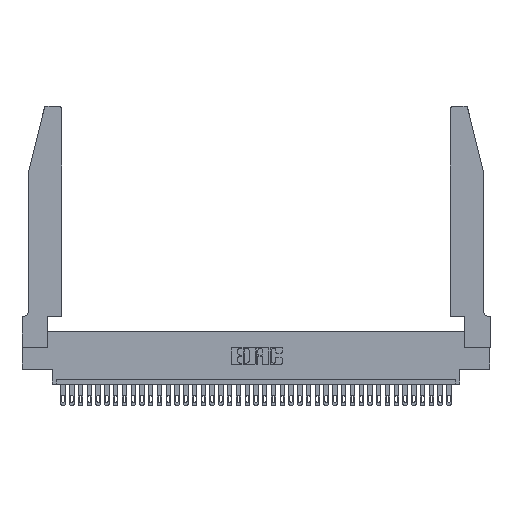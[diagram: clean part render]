
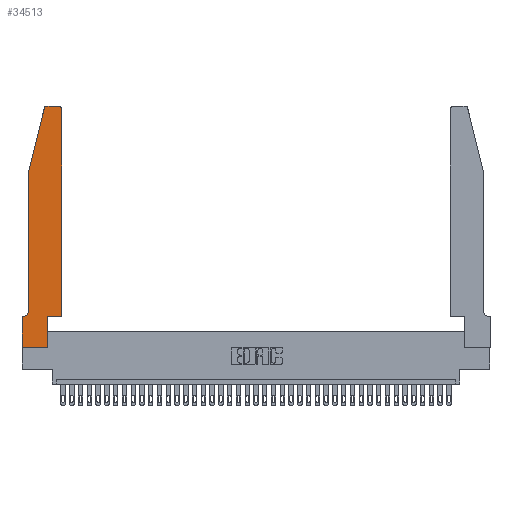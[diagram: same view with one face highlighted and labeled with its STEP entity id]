
A CAD part, top view. The second image highlights one B-rep face of the part: STEP entity #34513.
In plain terms, the highlighted planar face has unit normal (0, 0, 1).
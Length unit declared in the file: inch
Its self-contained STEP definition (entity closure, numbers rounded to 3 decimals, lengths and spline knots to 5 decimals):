
#97 = VERTEX_POINT ( 'NONE', #2483 ) ;
#175 = CARTESIAN_POINT ( 'NONE',  ( 0.0755, 2., 0.37 ) ) ;
#212 = CARTESIAN_POINT ( 'NONE',  ( 0.284, 2.72, 0.37 ) ) ;
#771 = VERTEX_POINT ( 'NONE', #37358 ) ;
#863 = CARTESIAN_POINT ( 'NONE',  ( 0.0755, 0.42, 0.37 ) ) ;
#1432 = EDGE_CURVE ( 'NONE', #24707, #26314, #30907, .T. ) ;
#2483 = CARTESIAN_POINT ( 'NONE',  ( 0.2865, 0.35, 0.37 ) ) ;
#2685 = EDGE_CURVE ( 'NONE', #26314, #23081, #18780, .T. ) ;
#3274 = ORIENTED_EDGE ( 'NONE', *, *, #8241, .T. ) ;
#3347 = CIRCLE ( 'NONE', #3746, 0.07 ) ;
#3746 = AXIS2_PLACEMENT_3D ( 'NONE', #6014, #6139, #11941 ) ;
#3758 = CARTESIAN_POINT ( 'NONE',  ( 0.2865, 0.35, 0.37 ) ) ;
#4425 = DIRECTION ( 'NONE',  ( 0., 1., 0. ) ) ;
#4665 = CARTESIAN_POINT ( 'NONE',  ( 0.4205, 2.75, 0.37 ) ) ;
#4867 = VERTEX_POINT ( 'NONE', #12759 ) ;
#5276 = CARTESIAN_POINT ( 'NONE',  ( 0., 0., 0.37 ) ) ;
#5482 = CARTESIAN_POINT ( 'NONE',  ( 0.25487, 2.72718, 0.37 ) ) ;
#6014 = CARTESIAN_POINT ( 'NONE',  ( 0.0055, 0.42, 0.37 ) ) ;
#6139 = DIRECTION ( 'NONE',  ( 0., 0., -1. ) ) ;
#6354 = VECTOR ( 'NONE', #14589, 39.37008 ) ;
#7670 = ORIENTED_EDGE ( 'NONE', *, *, #2685, .T. ) ;
#8241 = EDGE_CURVE ( 'NONE', #9883, #97, #9208, .T. ) ;
#8861 = ORIENTED_EDGE ( 'NONE', *, *, #19691, .T. ) ;
#9193 = DIRECTION ( 'NONE',  ( 0., 1., 0. ) ) ;
#9208 = LINE ( 'NONE', #3758, #34604 ) ;
#9423 = VECTOR ( 'NONE', #26111, 39.37008 ) ;
#9756 = ORIENTED_EDGE ( 'NONE', *, *, #19706, .T. ) ;
#9883 = VERTEX_POINT ( 'NONE', #12087 ) ;
#10145 = VECTOR ( 'NONE', #11916, 39.37008 ) ;
#10898 = DIRECTION ( 'NONE',  ( 0., 0., 1. ) ) ;
#11292 = CARTESIAN_POINT ( 'NONE',  ( 0.0755, 2., 0.37 ) ) ;
#11916 = DIRECTION ( 'NONE',  ( 0., -1., 0. ) ) ;
#11941 = DIRECTION ( 'NONE',  ( -1., 0., 0. ) ) ;
#12087 = CARTESIAN_POINT ( 'NONE',  ( 0.2865, 0., 0.37 ) ) ;
#12759 = CARTESIAN_POINT ( 'NONE',  ( 0., 0.35, 0.37 ) ) ;
#13321 = ORIENTED_EDGE ( 'NONE', *, *, #31277, .T. ) ;
#13360 = LINE ( 'NONE', #175, #10145 ) ;
#13736 = DIRECTION ( 'NONE',  ( 1., 0., 0. ) ) ;
#13812 = ORIENTED_EDGE ( 'NONE', *, *, #15193, .T. ) ;
#14589 = DIRECTION ( 'NONE',  ( 1., 0., 0. ) ) ;
#14702 = VERTEX_POINT ( 'NONE', #17727 ) ;
#14715 = FACE_OUTER_BOUND ( 'NONE', #21656, .T. ) ;
#15193 = EDGE_CURVE ( 'NONE', #23081, #16428, #13360, .T. ) ;
#15401 = CARTESIAN_POINT ( 'NONE',  ( 0., 0.35, 0.37 ) ) ;
#15605 = ORIENTED_EDGE ( 'NONE', *, *, #25438, .T. ) ;
#16428 = VERTEX_POINT ( 'NONE', #863 ) ;
#17727 = CARTESIAN_POINT ( 'NONE',  ( 0.0055, 0.35, 0.37 ) ) ;
#18396 = ORIENTED_EDGE ( 'NONE', *, *, #26589, .T. ) ;
#18499 = DIRECTION ( 'NONE',  ( 1., 0., 0. ) ) ;
#18740 = CARTESIAN_POINT ( 'NONE',  ( 0., 0., 0.37 ) ) ;
#18780 = LINE ( 'NONE', #23416, #28484 ) ;
#19011 = ORIENTED_EDGE ( 'NONE', *, *, #21983, .T. ) ;
#19507 = AXIS2_PLACEMENT_3D ( 'NONE', #15401, #24183, #30630 ) ;
#19691 = EDGE_CURVE ( 'NONE', #4867, #32729, #24784, .T. ) ;
#19706 = EDGE_CURVE ( 'NONE', #771, #23542, #29541, .T. ) ;
#20011 = CIRCLE ( 'NONE', #24924, 0.03 ) ;
#20039 = EDGE_CURVE ( 'NONE', #97, #771, #37313, .T. ) ;
#20171 = CARTESIAN_POINT ( 'NONE',  ( 0.2605, 2.75, 0.37 ) ) ;
#20582 = VECTOR ( 'NONE', #33196, 39.37008 ) ;
#20840 = ORIENTED_EDGE ( 'NONE', *, *, #1432, .T. ) ;
#20843 = DIRECTION ( 'NONE',  ( 0., 0., 1. ) ) ;
#20893 = DIRECTION ( 'NONE',  ( -1., 0., 0. ) ) ;
#21656 = EDGE_LOOP ( 'NONE', ( #24133, #20840, #7670, #13812, #15605, #13321, #8861, #18396, #3274, #23190, #9756, #19011 ) ) ;
#21983 = EDGE_CURVE ( 'NONE', #23542, #36411, #20011, .T. ) ;
#22531 = DIRECTION ( 'NONE',  ( 1., 0., 0. ) ) ;
#22753 = VECTOR ( 'NONE', #4425, 39.37008 ) ;
#23052 = AXIS2_PLACEMENT_3D ( 'NONE', #212, #20843, #13736 ) ;
#23081 = VERTEX_POINT ( 'NONE', #11292 ) ;
#23190 = ORIENTED_EDGE ( 'NONE', *, *, #20039, .T. ) ;
#23416 = CARTESIAN_POINT ( 'NONE',  ( 0.0755, 2., 0.37 ) ) ;
#23542 = VERTEX_POINT ( 'NONE', #31293 ) ;
#23772 = CARTESIAN_POINT ( 'NONE',  ( 0.0755, 0.35, 0.37 ) ) ;
#24133 = ORIENTED_EDGE ( 'NONE', *, *, #37195, .T. ) ;
#24183 = DIRECTION ( 'NONE',  ( 0., 0., 1. ) ) ;
#24187 = CARTESIAN_POINT ( 'NONE',  ( 0., 0., 0.37 ) ) ;
#24707 = VERTEX_POINT ( 'NONE', #29298 ) ;
#24784 = LINE ( 'NONE', #18740, #20582 ) ;
#24924 = AXIS2_PLACEMENT_3D ( 'NONE', #37011, #10898, #22531 ) ;
#25194 = CARTESIAN_POINT ( 'NONE',  ( 0.4505, 0.35, 0.37 ) ) ;
#25438 = EDGE_CURVE ( 'NONE', #16428, #14702, #3347, .T. ) ;
#26111 = DIRECTION ( 'NONE',  ( -1., 0., 0. ) ) ;
#26314 = VERTEX_POINT ( 'NONE', #5482 ) ;
#26589 = EDGE_CURVE ( 'NONE', #32729, #9883, #37219, .T. ) ;
#28484 = VECTOR ( 'NONE', #32083, 39.37008 ) ;
#29298 = CARTESIAN_POINT ( 'NONE',  ( 0.284, 2.75, 0.37 ) ) ;
#29347 = VECTOR ( 'NONE', #18499, 39.37008 ) ;
#29541 = LINE ( 'NONE', #25194, #22753 ) ;
#30630 = DIRECTION ( 'NONE',  ( 1., 0., 0. ) ) ;
#30907 = CIRCLE ( 'NONE', #23052, 0.03 ) ;
#31277 = EDGE_CURVE ( 'NONE', #14702, #4867, #33616, .T. ) ;
#31293 = CARTESIAN_POINT ( 'NONE',  ( 0.4505, 2.72, 0.37 ) ) ;
#32083 = DIRECTION ( 'NONE',  ( -0.239, -0.971, 0. ) ) ;
#32729 = VERTEX_POINT ( 'NONE', #5276 ) ;
#33196 = DIRECTION ( 'NONE',  ( 0., -1., 0. ) ) ;
#33616 = LINE ( 'NONE', #23772, #34054 ) ;
#33908 = LINE ( 'NONE', #20171, #9423 ) ;
#34054 = VECTOR ( 'NONE', #20893, 39.37008 ) ;
#34513 = ADVANCED_FACE ( 'NONE', ( #14715 ), #36050, .T. ) ;
#34604 = VECTOR ( 'NONE', #9193, 39.37008 ) ;
#35244 = CARTESIAN_POINT ( 'NONE',  ( 0.4505, 0.35, 0.37 ) ) ;
#36050 = PLANE ( 'NONE',  #19507 ) ;
#36411 = VERTEX_POINT ( 'NONE', #4665 ) ;
#37011 = CARTESIAN_POINT ( 'NONE',  ( 0.4205, 2.72, 0.37 ) ) ;
#37195 = EDGE_CURVE ( 'NONE', #36411, #24707, #33908, .T. ) ;
#37219 = LINE ( 'NONE', #24187, #29347 ) ;
#37313 = LINE ( 'NONE', #35244, #6354 ) ;
#37358 = CARTESIAN_POINT ( 'NONE',  ( 0.4505, 0.35, 0.37 ) ) ;
